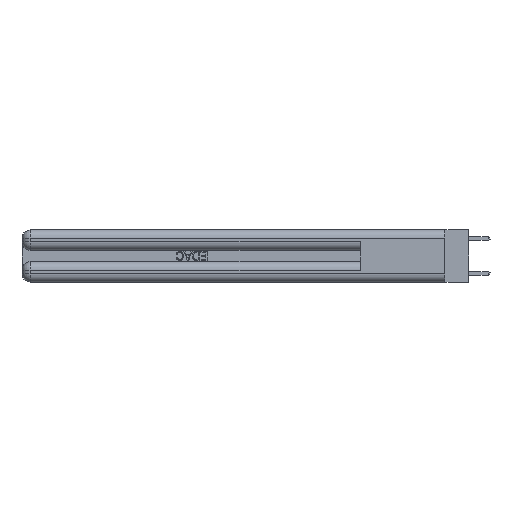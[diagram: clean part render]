
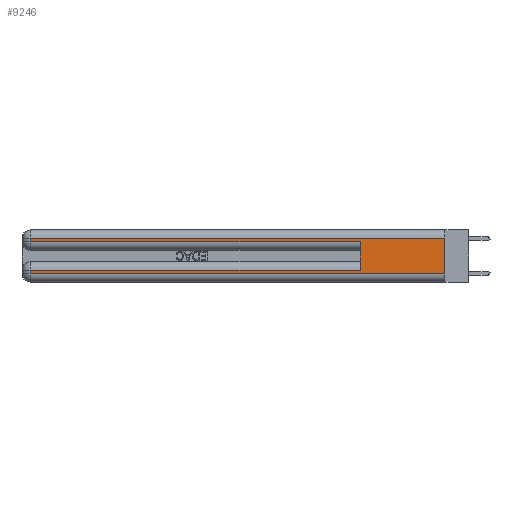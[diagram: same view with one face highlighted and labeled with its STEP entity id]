
A CAD part, left-side view. The second image highlights one B-rep face of the part: STEP entity #9246.
In plain terms, the highlighted planar face has unit normal (-1, 0, 0).
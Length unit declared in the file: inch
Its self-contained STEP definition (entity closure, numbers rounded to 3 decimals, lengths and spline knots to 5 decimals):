
#64 = CARTESIAN_POINT ( 'NONE',  ( 0., 2.94, 0.285 ) ) ;
#637 = CARTESIAN_POINT ( 'NONE',  ( 0., 0., 0.31 ) ) ;
#935 = LINE ( 'NONE', #6451, #20901 ) ;
#1064 = ORIENTED_EDGE ( 'NONE', *, *, #32861, .T. ) ;
#1250 = DIRECTION ( 'NONE',  ( 0., 1., 0. ) ) ;
#1422 = DIRECTION ( 'NONE',  ( 0., 0., -1. ) ) ;
#1439 = VECTOR ( 'NONE', #10329, 39.37008 ) ;
#1445 = EDGE_CURVE ( 'NONE', #21885, #17772, #20967, .T. ) ;
#3639 = DIRECTION ( 'NONE',  ( 0., 1., 0. ) ) ;
#4070 = VECTOR ( 'NONE', #1422, 39.37008 ) ;
#4522 = VERTEX_POINT ( 'NONE', #12251 ) ;
#5443 = CARTESIAN_POINT ( 'NONE',  ( 0., 0., 0.31 ) ) ;
#6291 = CARTESIAN_POINT ( 'NONE',  ( 0., 2.94, 0.37 ) ) ;
#6398 = DIRECTION ( 'NONE',  ( 0., 0., 1. ) ) ;
#6451 = CARTESIAN_POINT ( 'NONE',  ( 0., 0., 0.085 ) ) ;
#7853 = ORIENTED_EDGE ( 'NONE', *, *, #20581, .T. ) ;
#9115 = ORIENTED_EDGE ( 'NONE', *, *, #18620, .T. ) ;
#9246 = ADVANCED_FACE ( 'NONE', ( #14530 ), #18914, .F. ) ;
#9379 = LINE ( 'NONE', #24851, #18374 ) ;
#9493 = EDGE_CURVE ( 'NONE', #9560, #11517, #12115, .T. ) ;
#9560 = VERTEX_POINT ( 'NONE', #17822 ) ;
#9616 = CARTESIAN_POINT ( 'NONE',  ( 0., 2.94, 0.06 ) ) ;
#9945 = AXIS2_PLACEMENT_3D ( 'NONE', #27142, #11666, #24125 ) ;
#10329 = DIRECTION ( 'NONE',  ( 0., -1., 0. ) ) ;
#10452 = ORIENTED_EDGE ( 'NONE', *, *, #26378, .T. ) ;
#10754 = EDGE_CURVE ( 'NONE', #21981, #11517, #15880, .T. ) ;
#11517 = VERTEX_POINT ( 'NONE', #31707 ) ;
#11666 = DIRECTION ( 'NONE',  ( 1., 0., 0. ) ) ;
#11677 = ORIENTED_EDGE ( 'NONE', *, *, #1445, .T. ) ;
#11763 = VERTEX_POINT ( 'NONE', #24146 ) ;
#12115 = LINE ( 'NONE', #27418, #23039 ) ;
#12251 = CARTESIAN_POINT ( 'NONE',  ( 0., 2.94, 0.085 ) ) ;
#12338 = VERTEX_POINT ( 'NONE', #9616 ) ;
#12448 = EDGE_CURVE ( 'NONE', #21885, #11763, #26102, .T. ) ;
#13323 = CARTESIAN_POINT ( 'NONE',  ( 0., 0., 0.37 ) ) ;
#13641 = ORIENTED_EDGE ( 'NONE', *, *, #12448, .F. ) ;
#14530 = FACE_OUTER_BOUND ( 'NONE', #27513, .T. ) ;
#14562 = VECTOR ( 'NONE', #31301, 39.37008 ) ;
#15180 = VECTOR ( 'NONE', #30621, 39.37008 ) ;
#15501 = CARTESIAN_POINT ( 'NONE',  ( 0., 0., 0.06 ) ) ;
#15880 = LINE ( 'NONE', #26307, #1439 ) ;
#16306 = CARTESIAN_POINT ( 'NONE',  ( 0., 2.94, 0.31 ) ) ;
#16360 = VECTOR ( 'NONE', #3639, 39.37008 ) ;
#17772 = VERTEX_POINT ( 'NONE', #16306 ) ;
#17822 = CARTESIAN_POINT ( 'NONE',  ( 0., 0.6, 0.085 ) ) ;
#18374 = VECTOR ( 'NONE', #30408, 39.37008 ) ;
#18620 = EDGE_CURVE ( 'NONE', #4522, #12338, #9379, .T. ) ;
#18914 = PLANE ( 'NONE',  #9945 ) ;
#19835 = ORIENTED_EDGE ( 'NONE', *, *, #9493, .F. ) ;
#20532 = LINE ( 'NONE', #15501, #15180 ) ;
#20581 = EDGE_CURVE ( 'NONE', #12338, #11763, #20532, .T. ) ;
#20901 = VECTOR ( 'NONE', #1250, 39.37008 ) ;
#20967 = LINE ( 'NONE', #637, #16360 ) ;
#21885 = VERTEX_POINT ( 'NONE', #5443 ) ;
#21981 = VERTEX_POINT ( 'NONE', #64 ) ;
#23039 = VECTOR ( 'NONE', #6398, 39.37008 ) ;
#24125 = DIRECTION ( 'NONE',  ( 0., 0., -1. ) ) ;
#24146 = CARTESIAN_POINT ( 'NONE',  ( 0., 0., 0.06 ) ) ;
#24851 = CARTESIAN_POINT ( 'NONE',  ( 0., 2.94, 0.37 ) ) ;
#26016 = ORIENTED_EDGE ( 'NONE', *, *, #10754, .T. ) ;
#26102 = LINE ( 'NONE', #13323, #14562 ) ;
#26307 = CARTESIAN_POINT ( 'NONE',  ( 0., 0., 0.285 ) ) ;
#26378 = EDGE_CURVE ( 'NONE', #17772, #21981, #29184, .T. ) ;
#27142 = CARTESIAN_POINT ( 'NONE',  ( 0., 0., 0.37 ) ) ;
#27418 = CARTESIAN_POINT ( 'NONE',  ( 0., 0.6, 0.145 ) ) ;
#27513 = EDGE_LOOP ( 'NONE', ( #13641, #11677, #10452, #26016, #19835, #1064, #9115, #7853 ) ) ;
#29184 = LINE ( 'NONE', #6291, #4070 ) ;
#30408 = DIRECTION ( 'NONE',  ( 0., 0., -1. ) ) ;
#30621 = DIRECTION ( 'NONE',  ( 0., -1., 0. ) ) ;
#31301 = DIRECTION ( 'NONE',  ( 0., 0., -1. ) ) ;
#31707 = CARTESIAN_POINT ( 'NONE',  ( 0., 0.6, 0.285 ) ) ;
#32861 = EDGE_CURVE ( 'NONE', #9560, #4522, #935, .T. ) ;
